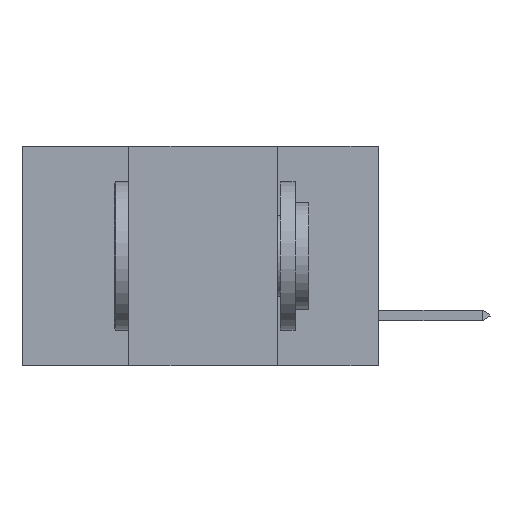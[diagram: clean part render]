
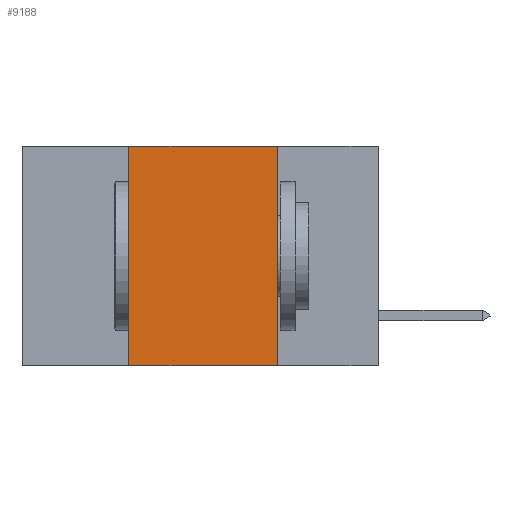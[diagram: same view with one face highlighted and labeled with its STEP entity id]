
A CAD part, left-side view. The second image highlights one B-rep face of the part: STEP entity #9188.
In plain terms, the highlighted planar face has unit normal (-1, 0, 0).
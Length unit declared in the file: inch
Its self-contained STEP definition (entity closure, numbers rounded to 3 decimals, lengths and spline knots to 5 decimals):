
#10 = AXIS2_PLACEMENT_3D ( 'NONE', #3522, #5473, #4330 ) ;
#157 = ORIENTED_EDGE ( 'NONE', *, *, #1351, .F. ) ;
#222 = VECTOR ( 'NONE', #8344, 39.37008 ) ;
#1300 = LINE ( 'NONE', #6469, #222 ) ;
#1351 = EDGE_CURVE ( 'NONE', #3575, #10479, #10485, .T. ) ;
#1550 = ORIENTED_EDGE ( 'NONE', *, *, #5704, .F. ) ;
#2090 = DIRECTION ( 'NONE',  ( 0., 0., -1. ) ) ;
#2854 = CARTESIAN_POINT ( 'NONE',  ( 0., 0.6, -0.37 ) ) ;
#3522 = CARTESIAN_POINT ( 'NONE',  ( 0., 0.6, 0. ) ) ;
#3575 = VERTEX_POINT ( 'NONE', #5969 ) ;
#3849 = VECTOR ( 'NONE', #6668, 39.37008 ) ;
#4185 = CARTESIAN_POINT ( 'NONE',  ( 0., 0.17, 0. ) ) ;
#4330 = DIRECTION ( 'NONE',  ( 0., 0., -1. ) ) ;
#5473 = DIRECTION ( 'NONE',  ( 1., 0., 0. ) ) ;
#5512 = ORIENTED_EDGE ( 'NONE', *, *, #10827, .F. ) ;
#5704 = EDGE_CURVE ( 'NONE', #11483, #3575, #1300, .T. ) ;
#5969 = CARTESIAN_POINT ( 'NONE',  ( 0., 0.17, 0. ) ) ;
#6465 = CARTESIAN_POINT ( 'NONE',  ( 0., 0.17, -0.37 ) ) ;
#6469 = CARTESIAN_POINT ( 'NONE',  ( 0., 0.6, 0. ) ) ;
#6484 = VECTOR ( 'NONE', #10582, 39.37008 ) ;
#6668 = DIRECTION ( 'NONE',  ( 0., -1., 0. ) ) ;
#6764 = EDGE_CURVE ( 'NONE', #11066, #10479, #7138, .T. ) ;
#6798 = CARTESIAN_POINT ( 'NONE',  ( 0., 0.42, 0. ) ) ;
#7106 = CARTESIAN_POINT ( 'NONE',  ( 0., 0.42, -0.37 ) ) ;
#7138 = LINE ( 'NONE', #2854, #3849 ) ;
#7809 = LINE ( 'NONE', #6798, #6484 ) ;
#7969 = ORIENTED_EDGE ( 'NONE', *, *, #6764, .T. ) ;
#8344 = DIRECTION ( 'NONE',  ( 0., -1., 0. ) ) ;
#9188 = ADVANCED_FACE ( 'NONE', ( #11612 ), #11233, .F. ) ;
#9721 = CARTESIAN_POINT ( 'NONE',  ( 0., 0.42, 0. ) ) ;
#10479 = VERTEX_POINT ( 'NONE', #6465 ) ;
#10485 = LINE ( 'NONE', #4185, #11563 ) ;
#10582 = DIRECTION ( 'NONE',  ( 0., 0., 1. ) ) ;
#10827 = EDGE_CURVE ( 'NONE', #11066, #11483, #7809, .T. ) ;
#11066 = VERTEX_POINT ( 'NONE', #7106 ) ;
#11095 = EDGE_LOOP ( 'NONE', ( #157, #1550, #5512, #7969 ) ) ;
#11233 = PLANE ( 'NONE',  #10 ) ;
#11483 = VERTEX_POINT ( 'NONE', #9721 ) ;
#11563 = VECTOR ( 'NONE', #2090, 39.37008 ) ;
#11612 = FACE_OUTER_BOUND ( 'NONE', #11095, .T. ) ;
